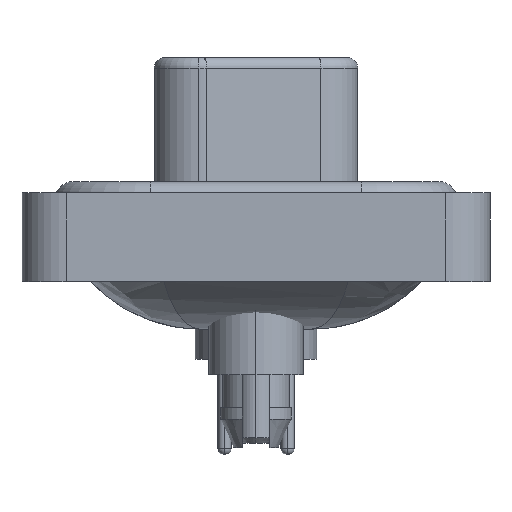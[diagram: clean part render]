
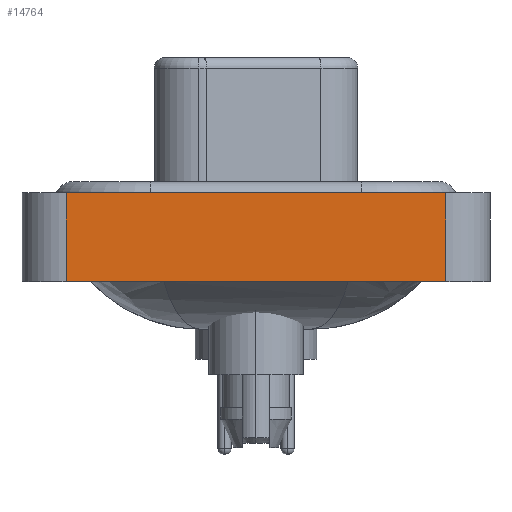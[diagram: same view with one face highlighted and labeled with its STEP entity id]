
A CAD part, left-side view. The second image highlights one B-rep face of the part: STEP entity #14764.
In plain terms, the highlighted planar face has unit normal (-1, 0, 0).
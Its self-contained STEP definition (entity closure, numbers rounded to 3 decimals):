
#242 = VECTOR ( 'NONE', #6092, 1000. ) ;
#373 = ORIENTED_EDGE ( 'NONE', *, *, #12234, .T. ) ;
#2091 = VERTEX_POINT ( 'NONE', #12321 ) ;
#2220 = LINE ( 'NONE', #3772, #6757 ) ;
#3024 = LINE ( 'NONE', #12985, #12610 ) ;
#3772 = CARTESIAN_POINT ( 'NONE',  ( -7.35, -8.55, -3.6 ) ) ;
#4012 = LINE ( 'NONE', #12661, #242 ) ;
#4512 = ORIENTED_EDGE ( 'NONE', *, *, #5233, .F. ) ;
#4623 = VERTEX_POINT ( 'NONE', #16840 ) ;
#4649 = CARTESIAN_POINT ( 'NONE',  ( -7.35, -8.55, -3.6 ) ) ;
#5233 = EDGE_CURVE ( 'NONE', #2091, #4623, #4012, .T. ) ;
#5385 = DIRECTION ( 'NONE',  ( 0., 0., 1. ) ) ;
#5795 = CARTESIAN_POINT ( 'NONE',  ( -7.35, -8.55, -3.6 ) ) ;
#5904 = DIRECTION ( 'NONE',  ( -1., 0., 0. ) ) ;
#6092 = DIRECTION ( 'NONE',  ( 0., -1., 0. ) ) ;
#6757 = VECTOR ( 'NONE', #9024, 1000. ) ;
#6802 = VECTOR ( 'NONE', #5385, 1000. ) ;
#7036 = CARTESIAN_POINT ( 'NONE',  ( -7.35, -8.55, -3.6 ) ) ;
#7654 = DIRECTION ( 'NONE',  ( 0., 0., 1. ) ) ;
#8023 = EDGE_CURVE ( 'NONE', #17194, #2091, #3024, .T. ) ;
#8260 = ORIENTED_EDGE ( 'NONE', *, *, #8023, .F. ) ;
#8287 = DIRECTION ( 'NONE',  ( 0., 0., 1. ) ) ;
#8988 = FACE_OUTER_BOUND ( 'NONE', #13928, .T. ) ;
#9024 = DIRECTION ( 'NONE',  ( 0., -1., 0. ) ) ;
#12216 = EDGE_CURVE ( 'NONE', #17194, #18403, #2220, .T. ) ;
#12234 = EDGE_CURVE ( 'NONE', #18403, #4623, #15347, .T. ) ;
#12321 = CARTESIAN_POINT ( 'NONE',  ( -7.35, 8.55, 0.4 ) ) ;
#12610 = VECTOR ( 'NONE', #8287, 1000. ) ;
#12661 = CARTESIAN_POINT ( 'NONE',  ( -7.35, -8.55, 0.4 ) ) ;
#12985 = CARTESIAN_POINT ( 'NONE',  ( -7.35, 8.55, -3.6 ) ) ;
#13928 = EDGE_LOOP ( 'NONE', ( #373, #4512, #8260, #21427 ) ) ;
#14764 = ADVANCED_FACE ( 'NONE', ( #8988 ), #20660, .T. ) ;
#15347 = LINE ( 'NONE', #7036, #6802 ) ;
#16840 = CARTESIAN_POINT ( 'NONE',  ( -7.35, -8.55, 0.4 ) ) ;
#17194 = VERTEX_POINT ( 'NONE', #19762 ) ;
#17221 = AXIS2_PLACEMENT_3D ( 'NONE', #5795, #5904, #7654 ) ;
#18403 = VERTEX_POINT ( 'NONE', #4649 ) ;
#19762 = CARTESIAN_POINT ( 'NONE',  ( -7.35, 8.55, -3.6 ) ) ;
#20660 = PLANE ( 'NONE',  #17221 ) ;
#21427 = ORIENTED_EDGE ( 'NONE', *, *, #12216, .T. ) ;
